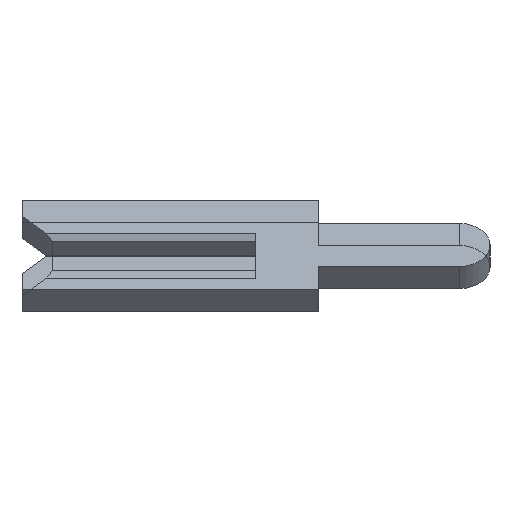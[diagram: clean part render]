
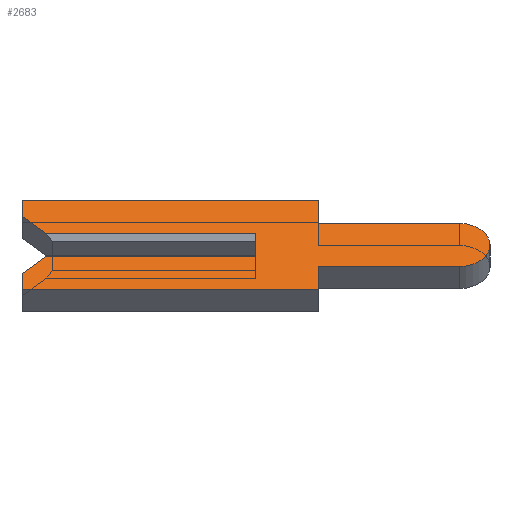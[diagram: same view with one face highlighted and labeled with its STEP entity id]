
A CAD part, left-side view. The second image highlights one B-rep face of the part: STEP entity #2683.
In plain terms, the highlighted face is planar.
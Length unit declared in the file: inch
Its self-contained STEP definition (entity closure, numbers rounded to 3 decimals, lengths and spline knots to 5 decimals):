
#86 = LINE ( 'NONE', #4052, #3291 ) ;
#91 = CARTESIAN_POINT ( 'NONE',  ( -0.01, -0.1305, -0.01 ) ) ;
#175 = EDGE_CURVE ( 'NONE', #3259, #1510, #3450, .T. ) ;
#207 = AXIS2_PLACEMENT_3D ( 'NONE', #3497, #3490, #4535 ) ;
#223 = ORIENTED_EDGE ( 'NONE', *, *, #2783, .F. ) ;
#243 = EDGE_CURVE ( 'NONE', #407, #2170, #86, .T. ) ;
#252 = EDGE_CURVE ( 'NONE', #1225, #1717, #822, .T. ) ;
#263 = CARTESIAN_POINT ( 'NONE',  ( -0.01, 0., 0.01 ) ) ;
#407 = VERTEX_POINT ( 'NONE', #2622 ) ;
#426 = VECTOR ( 'NONE', #677, 39.37008 ) ;
#535 = VECTOR ( 'NONE', #2787, 39.37008 ) ;
#661 = DIRECTION ( 'NONE',  ( 1., 0., 0. ) ) ;
#677 = DIRECTION ( 'NONE',  ( 0., -1., 0. ) ) ;
#692 = DIRECTION ( 'NONE',  ( 0., 1., 0. ) ) ;
#730 = EDGE_CURVE ( 'NONE', #3293, #1225, #1386, .T. ) ;
#822 = LINE ( 'NONE', #2437, #2651 ) ;
#841 = ORIENTED_EDGE ( 'NONE', *, *, #252, .F. ) ;
#876 = VECTOR ( 'NONE', #2819, 39.37008 ) ;
#885 = ORIENTED_EDGE ( 'NONE', *, *, #2254, .F. ) ;
#891 = ORIENTED_EDGE ( 'NONE', *, *, #3666, .F. ) ;
#964 = CARTESIAN_POINT ( 'NONE',  ( -0.01, -0.1305, 0.0195 ) ) ;
#976 = CARTESIAN_POINT ( 'NONE',  ( -0.01, 0.15, 0.026 ) ) ;
#981 = CARTESIAN_POINT ( 'NONE',  ( -0.01, 0., 0.0065 ) ) ;
#1038 = CARTESIAN_POINT ( 'NONE',  ( -0.01, 0.15, 0.04 ) ) ;
#1106 = LINE ( 'NONE', #2057, #876 ) ;
#1130 = ORIENTED_EDGE ( 'NONE', *, *, #2004, .F. ) ;
#1167 = DIRECTION ( 'NONE',  ( 0., -1., 0. ) ) ;
#1197 = ORIENTED_EDGE ( 'NONE', *, *, #3036, .T. ) ;
#1221 = VECTOR ( 'NONE', #2712, 39.37008 ) ;
#1225 = VERTEX_POINT ( 'NONE', #3793 ) ;
#1267 = EDGE_CURVE ( 'NONE', #3003, #1648, #1106, .T. ) ;
#1319 = PLANE ( 'NONE',  #207 ) ;
#1328 = VECTOR ( 'NONE', #692, 39.37008 ) ;
#1363 = CARTESIAN_POINT ( 'NONE',  ( -0.01, -0.04, 0.04 ) ) ;
#1377 = ORIENTED_EDGE ( 'NONE', *, *, #1267, .F. ) ;
#1381 = DIRECTION ( 'NONE',  ( 0., 0., -1. ) ) ;
#1386 = LINE ( 'NONE', #4446, #2496 ) ;
#1400 = DIRECTION ( 'NONE',  ( 0., 0., 1. ) ) ;
#1510 = VERTEX_POINT ( 'NONE', #1967 ) ;
#1559 = AXIS2_PLACEMENT_3D ( 'NONE', #2796, #661, #1381 ) ;
#1589 = CARTESIAN_POINT ( 'NONE',  ( -0.01, 0.15, -0.026 ) ) ;
#1594 = CIRCLE ( 'NONE', #1559, 0.0195 ) ;
#1648 = VERTEX_POINT ( 'NONE', #4155 ) ;
#1704 = CARTESIAN_POINT ( 'NONE',  ( -0.01, -0.04, -0.0195 ) ) ;
#1717 = VERTEX_POINT ( 'NONE', #1589 ) ;
#1855 = ORIENTED_EDGE ( 'NONE', *, *, #175, .F. ) ;
#1939 = LINE ( 'NONE', #1363, #4246 ) ;
#1967 = CARTESIAN_POINT ( 'NONE',  ( -0.01, 0., -0.01 ) ) ;
#1976 = CARTESIAN_POINT ( 'NONE',  ( -0.01, -0.1305, -0.0195 ) ) ;
#2004 = EDGE_CURVE ( 'NONE', #2710, #407, #1939, .T. ) ;
#2017 = DIRECTION ( 'NONE',  ( 0., 0., 1. ) ) ;
#2057 = CARTESIAN_POINT ( 'NONE',  ( -0.01, 0.1305, 0.0065 ) ) ;
#2106 = VECTOR ( 'NONE', #3047, 39.37008 ) ;
#2129 = CARTESIAN_POINT ( 'NONE',  ( -0.01, 0.134, -0.01 ) ) ;
#2164 = LINE ( 'NONE', #3514, #1328 ) ;
#2170 = VERTEX_POINT ( 'NONE', #964 ) ;
#2221 = VECTOR ( 'NONE', #2017, 39.37008 ) ;
#2254 = EDGE_CURVE ( 'NONE', #1510, #2552, #4415, .T. ) ;
#2315 = ORIENTED_EDGE ( 'NONE', *, *, #3915, .F. ) ;
#2333 = VECTOR ( 'NONE', #1167, 39.37008 ) ;
#2362 = VERTEX_POINT ( 'NONE', #1704 ) ;
#2412 = CARTESIAN_POINT ( 'NONE',  ( -0.01, 0.134, 0.01 ) ) ;
#2437 = CARTESIAN_POINT ( 'NONE',  ( -0.01, 0.15, -0.026 ) ) ;
#2496 = VECTOR ( 'NONE', #2694, 39.37008 ) ;
#2544 = LINE ( 'NONE', #2691, #535 ) ;
#2552 = VERTEX_POINT ( 'NONE', #263 ) ;
#2622 = CARTESIAN_POINT ( 'NONE',  ( -0.01, -0.04, 0.0195 ) ) ;
#2651 = VECTOR ( 'NONE', #1400, 39.37008 ) ;
#2683 = ADVANCED_FACE ( 'NONE', ( #4356 ), #1319, .F. ) ;
#2691 = CARTESIAN_POINT ( 'NONE',  ( -0.01, 0.1305, -0.0065 ) ) ;
#2694 = DIRECTION ( 'NONE',  ( 0., 1., 0. ) ) ;
#2704 = DIRECTION ( 'NONE',  ( 0., 0., 1. ) ) ;
#2710 = VERTEX_POINT ( 'NONE', #4220 ) ;
#2712 = DIRECTION ( 'NONE',  ( 0., -1., 0. ) ) ;
#2740 = ORIENTED_EDGE ( 'NONE', *, *, #243, .F. ) ;
#2765 = VECTOR ( 'NONE', #2704, 39.37008 ) ;
#2783 = EDGE_CURVE ( 'NONE', #3095, #2710, #3842, .T. ) ;
#2787 = DIRECTION ( 'NONE',  ( 0., -0.707, 0.707 ) ) ;
#2796 = CARTESIAN_POINT ( 'NONE',  ( -0.01, -0.1305, 0. ) ) ;
#2819 = DIRECTION ( 'NONE',  ( 0., 0.707, 0.707 ) ) ;
#2852 = ORIENTED_EDGE ( 'NONE', *, *, #4248, .F. ) ;
#2903 = CARTESIAN_POINT ( 'NONE',  ( -0.01, 0.15, 0.04 ) ) ;
#2938 = DIRECTION ( 'NONE',  ( 0., -1., 0. ) ) ;
#3003 = VERTEX_POINT ( 'NONE', #2412 ) ;
#3036 = EDGE_CURVE ( 'NONE', #3003, #2552, #3397, .T. ) ;
#3047 = DIRECTION ( 'NONE',  ( 0., 0., -1. ) ) ;
#3095 = VERTEX_POINT ( 'NONE', #1038 ) ;
#3259 = VERTEX_POINT ( 'NONE', #2129 ) ;
#3275 = EDGE_CURVE ( 'NONE', #3851, #2362, #2164, .T. ) ;
#3291 = VECTOR ( 'NONE', #2938, 39.37008 ) ;
#3293 = VERTEX_POINT ( 'NONE', #3530 ) ;
#3366 = EDGE_CURVE ( 'NONE', #2170, #3851, #1594, .T. ) ;
#3397 = LINE ( 'NONE', #3900, #426 ) ;
#3450 = LINE ( 'NONE', #91, #2333 ) ;
#3459 = DIRECTION ( 'NONE',  ( 0., 0., -1. ) ) ;
#3490 = DIRECTION ( 'NONE',  ( 1., 0., 0. ) ) ;
#3497 = CARTESIAN_POINT ( 'NONE',  ( -0.01, -0.1305, 0. ) ) ;
#3514 = CARTESIAN_POINT ( 'NONE',  ( -0.01, -0.04, -0.0195 ) ) ;
#3530 = CARTESIAN_POINT ( 'NONE',  ( -0.01, -0.04, -0.04 ) ) ;
#3651 = EDGE_LOOP ( 'NONE', ( #1197, #885, #1855, #2852, #841, #4358, #891, #4239, #3816, #2740, #1130, #223, #2315, #1377 ) ) ;
#3666 = EDGE_CURVE ( 'NONE', #2362, #3293, #4128, .T. ) ;
#3793 = CARTESIAN_POINT ( 'NONE',  ( -0.01, 0.15, -0.04 ) ) ;
#3814 = CARTESIAN_POINT ( 'NONE',  ( -0.01, -0.04, -0.04 ) ) ;
#3816 = ORIENTED_EDGE ( 'NONE', *, *, #3366, .F. ) ;
#3842 = LINE ( 'NONE', #2903, #1221 ) ;
#3851 = VERTEX_POINT ( 'NONE', #1976 ) ;
#3900 = CARTESIAN_POINT ( 'NONE',  ( -0.01, 0.15, 0.01 ) ) ;
#3915 = EDGE_CURVE ( 'NONE', #1648, #3095, #4469, .T. ) ;
#4052 = CARTESIAN_POINT ( 'NONE',  ( -0.01, -0.04, 0.0195 ) ) ;
#4128 = LINE ( 'NONE', #3814, #2106 ) ;
#4155 = CARTESIAN_POINT ( 'NONE',  ( -0.01, 0.15, 0.026 ) ) ;
#4220 = CARTESIAN_POINT ( 'NONE',  ( -0.01, -0.04, 0.04 ) ) ;
#4239 = ORIENTED_EDGE ( 'NONE', *, *, #3275, .F. ) ;
#4246 = VECTOR ( 'NONE', #3459, 39.37008 ) ;
#4248 = EDGE_CURVE ( 'NONE', #1717, #3259, #2544, .T. ) ;
#4356 = FACE_OUTER_BOUND ( 'NONE', #3651, .T. ) ;
#4358 = ORIENTED_EDGE ( 'NONE', *, *, #730, .F. ) ;
#4415 = LINE ( 'NONE', #981, #2221 ) ;
#4446 = CARTESIAN_POINT ( 'NONE',  ( -0.01, 0.15, -0.04 ) ) ;
#4469 = LINE ( 'NONE', #976, #2765 ) ;
#4535 = DIRECTION ( 'NONE',  ( 0., 0., -1. ) ) ;
